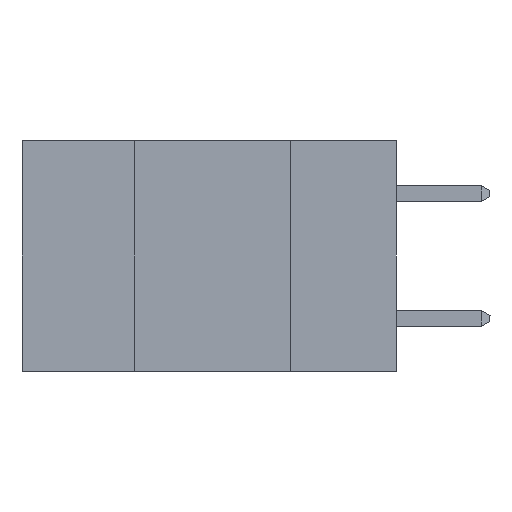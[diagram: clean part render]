
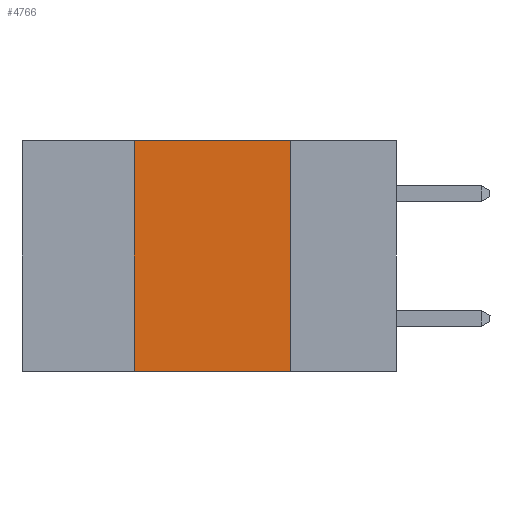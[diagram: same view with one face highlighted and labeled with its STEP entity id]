
A CAD part, left-side view. The second image highlights one B-rep face of the part: STEP entity #4766.
In plain terms, the highlighted planar face has unit normal (-1, 0, 0).
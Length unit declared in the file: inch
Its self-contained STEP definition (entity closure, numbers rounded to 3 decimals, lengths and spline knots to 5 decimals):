
#29 = CARTESIAN_POINT ( 'NONE',  ( 0., 0.6, 0. ) ) ;
#146 = EDGE_LOOP ( 'NONE', ( #9155, #7140, #1191, #270 ) ) ;
#270 = ORIENTED_EDGE ( 'NONE', *, *, #9512, .T. ) ;
#537 = DIRECTION ( 'NONE',  ( 1., 0., 0. ) ) ;
#1191 = ORIENTED_EDGE ( 'NONE', *, *, #6951, .F. ) ;
#1489 = VECTOR ( 'NONE', #7608, 39.37008 ) ;
#1589 = LINE ( 'NONE', #7672, #3411 ) ;
#2137 = CARTESIAN_POINT ( 'NONE',  ( 0., 0.42, -0.37 ) ) ;
#2209 = LINE ( 'NONE', #29, #7979 ) ;
#2406 = DIRECTION ( 'NONE',  ( 0., -1., 0. ) ) ;
#2746 = VECTOR ( 'NONE', #8469, 39.37008 ) ;
#2925 = CARTESIAN_POINT ( 'NONE',  ( 0., 0.6, 0. ) ) ;
#2937 = PLANE ( 'NONE',  #4079 ) ;
#3411 = VECTOR ( 'NONE', #2406, 39.37008 ) ;
#3522 = CARTESIAN_POINT ( 'NONE',  ( 0., 0.42, 0. ) ) ;
#3578 = CARTESIAN_POINT ( 'NONE',  ( 0., 0.17, -0.37 ) ) ;
#3832 = CARTESIAN_POINT ( 'NONE',  ( 0., 0.17, 0. ) ) ;
#4053 = VERTEX_POINT ( 'NONE', #3522 ) ;
#4079 = AXIS2_PLACEMENT_3D ( 'NONE', #2925, #537, #5338 ) ;
#4184 = FACE_OUTER_BOUND ( 'NONE', #146, .T. ) ;
#4592 = VERTEX_POINT ( 'NONE', #2137 ) ;
#4709 = DIRECTION ( 'NONE',  ( 0., -1., 0. ) ) ;
#4766 = ADVANCED_FACE ( 'NONE', ( #4184 ), #2937, .F. ) ;
#4890 = LINE ( 'NONE', #8985, #1489 ) ;
#5338 = DIRECTION ( 'NONE',  ( 0., 0., -1. ) ) ;
#6291 = CARTESIAN_POINT ( 'NONE',  ( 0., 0.42, -0.37 ) ) ;
#6951 = EDGE_CURVE ( 'NONE', #4592, #4053, #8675, .T. ) ;
#7140 = ORIENTED_EDGE ( 'NONE', *, *, #8668, .F. ) ;
#7608 = DIRECTION ( 'NONE',  ( 0., 0., -1. ) ) ;
#7672 = CARTESIAN_POINT ( 'NONE',  ( 0., 0.6, -0.37 ) ) ;
#7979 = VECTOR ( 'NONE', #4709, 39.37008 ) ;
#7981 = EDGE_CURVE ( 'NONE', #9454, #8382, #4890, .T. ) ;
#8382 = VERTEX_POINT ( 'NONE', #3578 ) ;
#8469 = DIRECTION ( 'NONE',  ( 0., 0., 1. ) ) ;
#8668 = EDGE_CURVE ( 'NONE', #4053, #9454, #2209, .T. ) ;
#8675 = LINE ( 'NONE', #6291, #2746 ) ;
#8985 = CARTESIAN_POINT ( 'NONE',  ( 0., 0.17, -0.37 ) ) ;
#9155 = ORIENTED_EDGE ( 'NONE', *, *, #7981, .F. ) ;
#9454 = VERTEX_POINT ( 'NONE', #3832 ) ;
#9512 = EDGE_CURVE ( 'NONE', #4592, #8382, #1589, .T. ) ;
